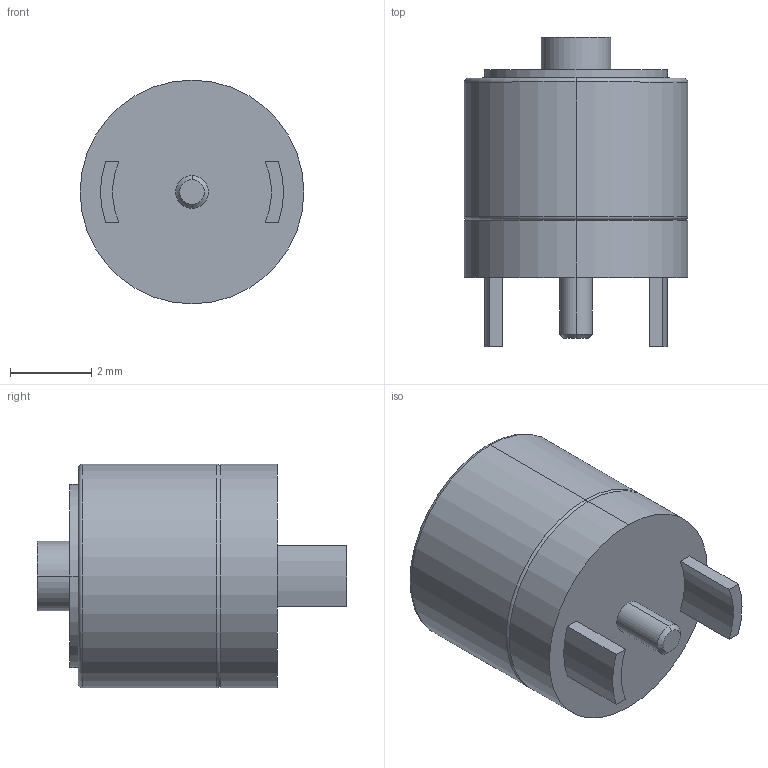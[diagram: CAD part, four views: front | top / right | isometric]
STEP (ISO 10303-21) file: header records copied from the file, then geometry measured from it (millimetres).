
FILE_DESCRIPTION (( 'STEP AP214' ), '1' );
FILE_NAME ('686A02222011A1E.STEP', '2023-04-26T14:27:43', ( '' ), ( '' ), 'SwSTEP 2.0', 'SolidWorks 2020', '' );
FILE_SCHEMA (( 'AUTOMOTIVE_DESIGN' ));
Length unit declared in the file: millimetre
Products named in the file (1): 686A02222011A1E
Bounding box: 5.5 x 7.6 x 5.5 mm (x, y, z)
Volume: 121.9 mm3; surface area: 219.3 mm2
Topology: 1 solids, 2 shells, 52 faces, 108 edges, 67 vertices
Faces by surface type: cylinder 22, plane 16, torus 8, cone 6
Entity records: 1996 total; most frequent: DIRECTION 278, CARTESIAN_POINT 226, ORIENTED_EDGE 212, AXIS2_PLACEMENT_3D 119, EDGE_CURVE 106, VERTEX_POINT 67, CIRCLE 66, EDGE_LOOP 63
